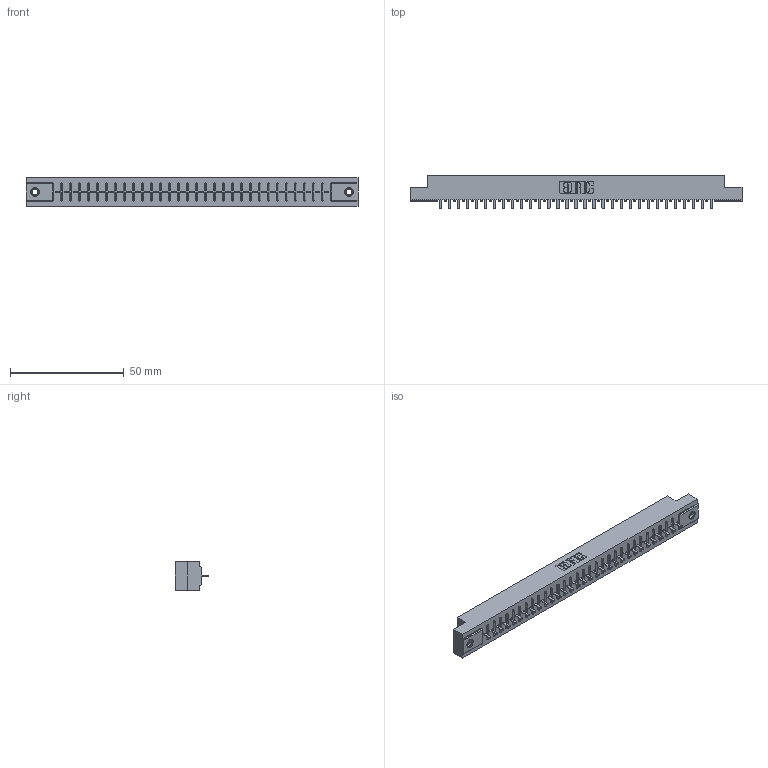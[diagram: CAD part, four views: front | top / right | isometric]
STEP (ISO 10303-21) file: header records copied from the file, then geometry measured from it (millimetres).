
FILE_DESCRIPTION (( 'STEP AP203' ), '1' );
FILE_NAME ('356-031-421-107.STEP', '2020-09-23T20:59:16', ( '' ), ( '' ), 'SwSTEP 2.0', 'SolidWorks 2020', '' );
FILE_SCHEMA (( 'CONFIG_CONTROL_DESIGN' ));
Length unit declared in the file: inch
Products named in the file (4): 306-290-001_121; 306 Part_.156 Dia; 356-031-421-107; 345-250-001_345-250-005-103
Assembly tree (34 placements, depth 2):
  356-031-421-107
    306 Part_.156 Dia
    306-290-001_121  x31
    345-250-001_345-250-005-103  x2
Bounding box: 145.85 x 14.88 x 12.7 mm (x, y, z)
Volume: 15972.6 mm3; surface area: 16088.4 mm2
Topology: 34 solids, 34 shells, 2346 faces, 6559 edges, 4198 vertices
Faces by surface type: plane 1557, cylinder 649, sphere 124, cone 12, torus 4
Entity records: 31475 total; most frequent: CARTESIAN_POINT 5263, ORIENTED_EDGE 5210, DIRECTION 5199, EDGE_CURVE 2605, VECTOR 2031, LINE 2031, VERTEX_POINT 1648, AXIS2_PLACEMENT_3D 1584
